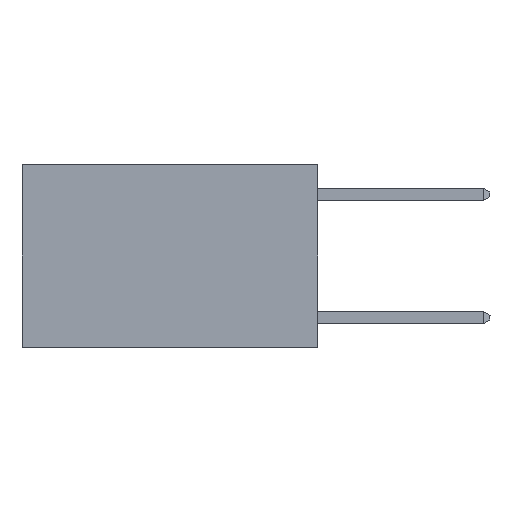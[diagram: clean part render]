
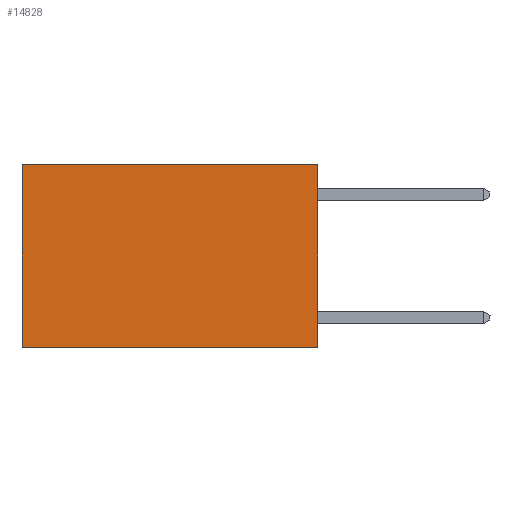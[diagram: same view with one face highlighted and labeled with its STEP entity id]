
A CAD part, left-side view. The second image highlights one B-rep face of the part: STEP entity #14828.
In plain terms, the highlighted planar face has unit normal (-1, 0, 0).
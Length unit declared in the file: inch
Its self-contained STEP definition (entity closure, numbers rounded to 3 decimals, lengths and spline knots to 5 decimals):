
#67 = LINE ( 'NONE', #5956, #10822 ) ;
#371 = DIRECTION ( 'NONE',  ( 0., 0., -1. ) ) ;
#757 = LINE ( 'NONE', #11158, #4781 ) ;
#1118 = LINE ( 'NONE', #5793, #3853 ) ;
#1561 = LINE ( 'NONE', #12974, #15425 ) ;
#1668 = PLANE ( 'NONE',  #9996 ) ;
#1927 = VERTEX_POINT ( 'NONE', #14398 ) ;
#2238 = VERTEX_POINT ( 'NONE', #16148 ) ;
#2258 = VERTEX_POINT ( 'NONE', #13978 ) ;
#2354 = EDGE_CURVE ( 'NONE', #2238, #1927, #1118, .T. ) ;
#2449 = ORIENTED_EDGE ( 'NONE', *, *, #12807, .F. ) ;
#3037 = CARTESIAN_POINT ( 'NONE',  ( 0.2625, 0., 0. ) ) ;
#3215 = ORIENTED_EDGE ( 'NONE', *, *, #13717, .F. ) ;
#3853 = VECTOR ( 'NONE', #15297, 39.37008 ) ;
#4388 = DIRECTION ( 'NONE',  ( 0., 0., -1. ) ) ;
#4781 = VECTOR ( 'NONE', #371, 39.37008 ) ;
#4956 = DIRECTION ( 'NONE',  ( 0., 1., 0. ) ) ;
#5793 = CARTESIAN_POINT ( 'NONE',  ( 0.2625, 0., 0. ) ) ;
#5956 = CARTESIAN_POINT ( 'NONE',  ( 0.2625, 0.6, 0. ) ) ;
#6146 = CARTESIAN_POINT ( 'NONE',  ( 0.2625, 0.6, -0.37 ) ) ;
#6610 = EDGE_LOOP ( 'NONE', ( #9730, #3215, #2449, #7041 ) ) ;
#7027 = EDGE_CURVE ( 'NONE', #1927, #16841, #67, .T. ) ;
#7041 = ORIENTED_EDGE ( 'NONE', *, *, #2354, .T. ) ;
#9730 = ORIENTED_EDGE ( 'NONE', *, *, #7027, .T. ) ;
#9996 = AXIS2_PLACEMENT_3D ( 'NONE', #3037, #12411, #4388 ) ;
#10822 = VECTOR ( 'NONE', #13985, 39.37008 ) ;
#11158 = CARTESIAN_POINT ( 'NONE',  ( 0.2625, 0., 0. ) ) ;
#12411 = DIRECTION ( 'NONE',  ( 1., 0., 0. ) ) ;
#12688 = FACE_OUTER_BOUND ( 'NONE', #6610, .T. ) ;
#12807 = EDGE_CURVE ( 'NONE', #2238, #2258, #757, .T. ) ;
#12974 = CARTESIAN_POINT ( 'NONE',  ( 0.2625, 0., -0.37 ) ) ;
#13717 = EDGE_CURVE ( 'NONE', #2258, #16841, #1561, .T. ) ;
#13978 = CARTESIAN_POINT ( 'NONE',  ( 0.2625, 0., -0.37 ) ) ;
#13985 = DIRECTION ( 'NONE',  ( 0., 0., -1. ) ) ;
#14398 = CARTESIAN_POINT ( 'NONE',  ( 0.2625, 0.6, 0. ) ) ;
#14828 = ADVANCED_FACE ( 'NONE', ( #12688 ), #1668, .F. ) ;
#15297 = DIRECTION ( 'NONE',  ( 0., 1., 0. ) ) ;
#15425 = VECTOR ( 'NONE', #4956, 39.37008 ) ;
#16148 = CARTESIAN_POINT ( 'NONE',  ( 0.2625, 0., 0. ) ) ;
#16841 = VERTEX_POINT ( 'NONE', #6146 ) ;
